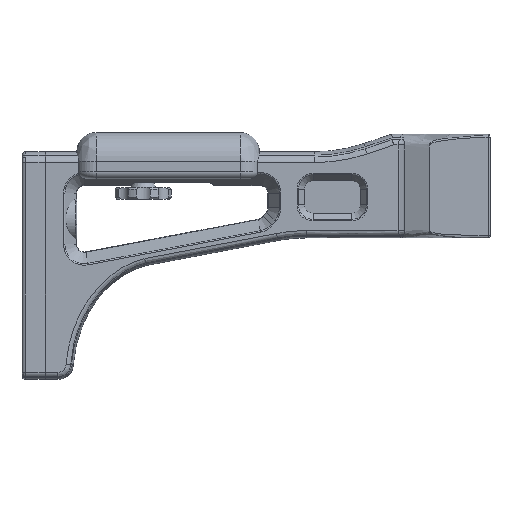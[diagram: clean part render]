
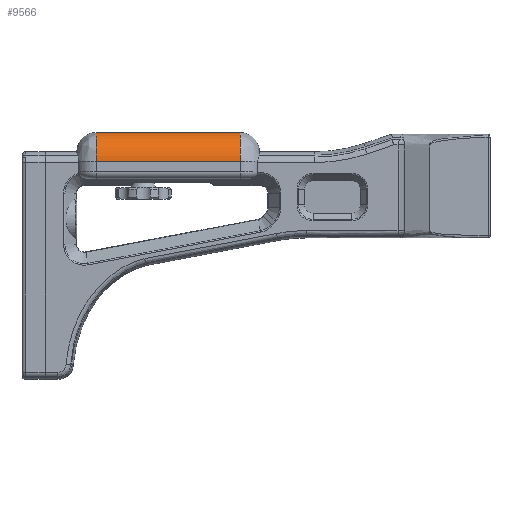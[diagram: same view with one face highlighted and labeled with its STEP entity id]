
A CAD part, top view. The second image highlights one B-rep face of the part: STEP entity #9566.
In plain terms, the highlighted cylindrical face has radius 15 mm (diameter 30 mm), a partial arc.
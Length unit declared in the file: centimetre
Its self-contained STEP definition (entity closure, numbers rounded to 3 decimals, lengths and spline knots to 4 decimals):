
#1035=LINE($,#24027,#1737);
#1037=LINE($,#24031,#1739);
#1737=VECTOR($,#12939,7.5);
#1739=VECTOR($,#12943,7.5);
#2807=FACE_OUTER_BOUND($,#3423,.T.);
#3423=EDGE_LOOP($,(#8797,#8798,#8799,#8800));
#3840=CIRCLE($,#10474,1.5);
#3843=CIRCLE($,#10481,1.5);
#4676=VERTEX_POINT($,#23929);
#4679=VERTEX_POINT($,#23936);
#4690=VERTEX_POINT($,#24026);
#4691=VERTEX_POINT($,#24030);
#6063=EDGE_CURVE($,#4679,#4676,#3840,.T.);
#6072=EDGE_CURVE($,#4690,#4676,#1035,.T.);
#6074=EDGE_CURVE($,#4679,#4691,#1037,.T.);
#6075=EDGE_CURVE($,#4690,#4691,#3843,.T.);
#8797=ORIENTED_EDGE($,*,*,#6074,.T.);
#8798=ORIENTED_EDGE($,*,*,#6075,.F.);
#8799=ORIENTED_EDGE($,*,*,#6072,.T.);
#8800=ORIENTED_EDGE($,*,*,#6063,.F.);
#9010=CYLINDRICAL_SURFACE($,#10480,1.5);
#9566=ADVANCED_FACE($,(#2807),#9010,.T.);
#10474=AXIS2_PLACEMENT_3D($,#23992,#12924,#12925);
#10480=AXIS2_PLACEMENT_3D($,#24029,#12941,#12942);
#10481=AXIS2_PLACEMENT_3D($,#24032,#12944,#12945);
#12924=DIRECTION('center_axis',(1.,0.,0.));
#12925=DIRECTION('ref_axis',(0.,0.707,0.707));
#12939=DIRECTION($,(1.,0.,0.));
#12941=DIRECTION('center_axis',(-1.,0.,0.));
#12942=DIRECTION('ref_axis',(0.,0.707,0.707));
#12943=DIRECTION($,(-1.,0.,0.));
#12944=DIRECTION('center_axis',(-1.,0.,0.));
#12945=DIRECTION('ref_axis',(0.,0.707,0.707));
#23929=CARTESIAN_POINT('',(-36.1912,3.8589,1.7723));
#23936=CARTESIAN_POINT('',(-36.1912,5.3589,0.2723));
#23992=CARTESIAN_POINT('Origin',(-36.1912,3.8589,0.2723));
#24026=CARTESIAN_POINT('',(-43.6912,3.8589,1.7723));
#24027=CARTESIAN_POINT($,(-43.8912,3.8589,1.7723));
#24029=CARTESIAN_POINT('Origin',(-43.3912,3.8589,0.2723));
#24030=CARTESIAN_POINT('',(-43.6912,5.3589,0.2723));
#24031=CARTESIAN_POINT($,(-43.3912,5.3589,0.2723));
#24032=CARTESIAN_POINT('Origin',(-43.6912,3.8589,0.2723));
